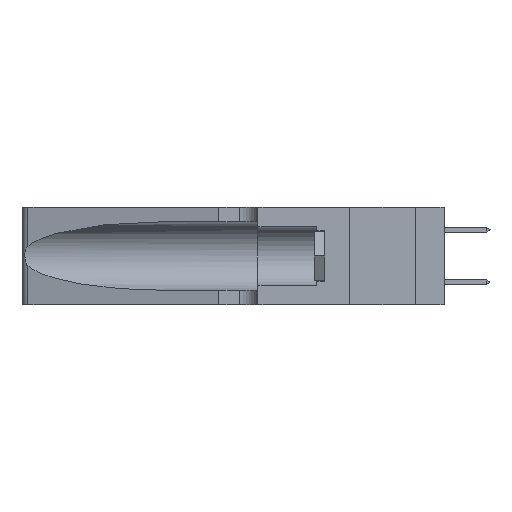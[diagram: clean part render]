
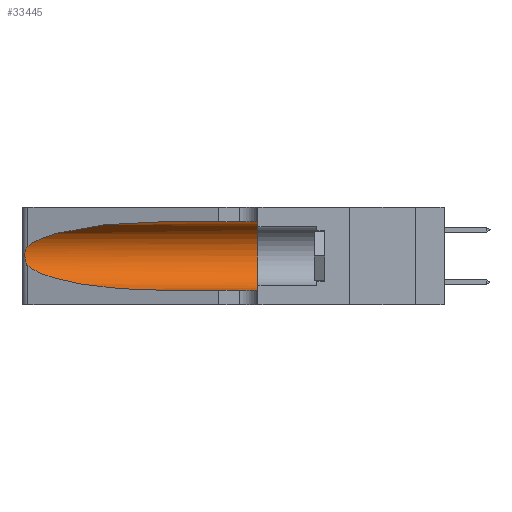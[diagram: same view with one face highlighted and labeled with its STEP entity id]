
A CAD part, left-side view. The second image highlights one B-rep face of the part: STEP entity #33445.
In plain terms, the highlighted cylindrical face has radius 3.308 mm (diameter 6.617 mm), a partial arc.
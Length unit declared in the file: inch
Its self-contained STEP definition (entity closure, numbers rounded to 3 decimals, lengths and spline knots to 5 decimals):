
#1452 = EDGE_LOOP ( 'NONE', ( #8038, #8470, #39785, #21762, #18273, #25114 ) ) ;
#2184 = CARTESIAN_POINT ( 'NONE',  ( 0.1305, 0.72297, 0.05475 ) ) ;
#2196 = CARTESIAN_POINT ( 'NONE',  ( 0.26018, 1.23835, 0.19895 ) ) ;
#3761 = VECTOR ( 'NONE', #10321, 39.37008 ) ;
#4998 = CARTESIAN_POINT ( 'NONE',  ( 0.25487, 1.22718, 0.14631 ) ) ;
#6235 = DIRECTION ( 'NONE',  ( 0., -1., 0. ) ) ;
#6544 = CARTESIAN_POINT ( 'NONE',  ( 0.25487, 1.22718, 0.22369 ) ) ;
#6580 = EDGE_CURVE ( 'NONE', #37651, #11041, #28170, .T. ) ;
#7029 = AXIS2_PLACEMENT_3D ( 'NONE', #22305, #6235, #38997 ) ;
#8038 = ORIENTED_EDGE ( 'NONE', *, *, #25024, .T. ) ;
#8470 = ORIENTED_EDGE ( 'NONE', *, *, #18121, .T. ) ;
#9690 = DIRECTION ( 'NONE',  ( 0., 1., 0. ) ) ;
#10237 = DIRECTION ( 'NONE',  ( 0., -1., 0. ) ) ;
#10321 = DIRECTION ( 'NONE',  ( 0., -1., 0. ) ) ;
#10370 = LINE ( 'NONE', #23724, #3761 ) ;
#11041 = VERTEX_POINT ( 'NONE', #36313 ) ;
#11594 = CARTESIAN_POINT ( 'NONE',  ( 0.18966, 0.96281, 0.31525 ) ) ;
#11728 = CARTESIAN_POINT ( 'NONE',  ( 0.2373, 1.15595, 0.28018 ) ) ;
#12830 = CARTESIAN_POINT ( 'NONE',  ( 0.25639, 1.23186, 0.15144 ) ) ;
#13076 = CARTESIAN_POINT ( 'NONE',  ( 0.1305, 0.35, 0.31525 ) ) ;
#13471 = CARTESIAN_POINT ( 'NONE',  ( 0.25487, 1.22718, 0.14631 ) ) ;
#14084 = CARTESIAN_POINT ( 'NONE',  ( 0.1305, 0.72297, 0.31525 ) ) ;
#14651 = VERTEX_POINT ( 'NONE', #14084 ) ;
#14954 = CARTESIAN_POINT ( 'NONE',  ( 0.25555, 1.22994, 0.2215 ) ) ;
#16225 = CARTESIAN_POINT ( 'NONE',  ( 0.25856, 1.23593, 0.16098 ) ) ;
#16981 =( BOUNDED_CURVE ( )  B_SPLINE_CURVE ( 3, ( #33908, #11594, #11728, #18089 ),
 .UNSPECIFIED., .F., .F. ) 
 B_SPLINE_CURVE_WITH_KNOTS ( ( 4, 4 ),
 ( 1.5708, 2.84003 ),
 .UNSPECIFIED. ) 
 CURVE ( )  GEOMETRIC_REPRESENTATION_ITEM ( )  RATIONAL_B_SPLINE_CURVE ( ( 1., 0.87, 0.87, 1. ) ) 
 REPRESENTATION_ITEM ( '' )  );
#18089 = CARTESIAN_POINT ( 'NONE',  ( 0.25487, 1.22718, 0.22369 ) ) ;
#18121 = EDGE_CURVE ( 'NONE', #35919, #19754, #18804, .T. ) ;
#18208 = CARTESIAN_POINT ( 'NONE',  ( 0.25787, 1.23484, 0.2124 ) ) ;
#18270 = EDGE_CURVE ( 'NONE', #24369, #11041, #10370, .T. ) ;
#18273 = ORIENTED_EDGE ( 'NONE', *, *, #6580, .F. ) ;
#18804 = B_SPLINE_CURVE_WITH_KNOTS ( 'NONE', 3,
 ( #31064, #14954, #37580, #18208, #40958, #2196, #31345, #25821, #38545, #16225, #22707, #12830, #29190, #32452 ),
 .UNSPECIFIED., .F., .F.,
 ( 4, 2, 2, 2, 2, 2, 4 ),
 ( 0., 0.00027, 0.00053, 0.00107, 0.0016, 0.00187, 0.00214 ),
 .UNSPECIFIED. ) ;
#19673 = LINE ( 'NONE', #20536, #27769 ) ;
#19754 = VERTEX_POINT ( 'NONE', #13471 ) ;
#20098 =( BOUNDED_CURVE ( )  B_SPLINE_CURVE ( 3, ( #4998, #21510, #24915, #28138 ),
 .UNSPECIFIED., .F., .T. ) 
 B_SPLINE_CURVE_WITH_KNOTS ( ( 4, 4 ),
 ( 3.44316, 4.71239 ),
 .UNSPECIFIED. ) 
 CURVE ( )  GEOMETRIC_REPRESENTATION_ITEM ( )  RATIONAL_B_SPLINE_CURVE ( ( 1., 0.87, 0.87, 1. ) ) 
 REPRESENTATION_ITEM ( '' )  );
#20536 = CARTESIAN_POINT ( 'NONE',  ( 0.1305, 1.61858, 0.31525 ) ) ;
#21410 = AXIS2_PLACEMENT_3D ( 'NONE', #28442, #9690, #40862 ) ;
#21510 = CARTESIAN_POINT ( 'NONE',  ( 0.2373, 1.15595, 0.08982 ) ) ;
#21762 = ORIENTED_EDGE ( 'NONE', *, *, #18270, .T. ) ;
#22305 = CARTESIAN_POINT ( 'NONE',  ( 0.1305, 1.61858, 0.185 ) ) ;
#22329 = EDGE_CURVE ( 'NONE', #19754, #24369, #20098, .T. ) ;
#22707 = CARTESIAN_POINT ( 'NONE',  ( 0.25789, 1.23486, 0.15765 ) ) ;
#23724 = CARTESIAN_POINT ( 'NONE',  ( 0.1305, 1.61858, 0.05475 ) ) ;
#24369 = VERTEX_POINT ( 'NONE', #2184 ) ;
#24915 = CARTESIAN_POINT ( 'NONE',  ( 0.18966, 0.96281, 0.05475 ) ) ;
#25024 = EDGE_CURVE ( 'NONE', #14651, #35919, #16981, .T. ) ;
#25114 = ORIENTED_EDGE ( 'NONE', *, *, #26198, .F. ) ;
#25821 = CARTESIAN_POINT ( 'NONE',  ( 0.26075, 1.23896, 0.178 ) ) ;
#26198 = EDGE_CURVE ( 'NONE', #14651, #37651, #19673, .T. ) ;
#27769 = VECTOR ( 'NONE', #10237, 39.37008 ) ;
#28138 = CARTESIAN_POINT ( 'NONE',  ( 0.1305, 0.72297, 0.05475 ) ) ;
#28170 = CIRCLE ( 'NONE', #21410, 0.13025 ) ;
#28442 = CARTESIAN_POINT ( 'NONE',  ( 0.1305, 0.35, 0.185 ) ) ;
#29190 = CARTESIAN_POINT ( 'NONE',  ( 0.25555, 1.22993, 0.14849 ) ) ;
#29606 = CYLINDRICAL_SURFACE ( 'NONE', #7029, 0.13025 ) ;
#31064 = CARTESIAN_POINT ( 'NONE',  ( 0.25487, 1.22718, 0.22369 ) ) ;
#31345 = CARTESIAN_POINT ( 'NONE',  ( 0.26075, 1.23896, 0.19203 ) ) ;
#32452 = CARTESIAN_POINT ( 'NONE',  ( 0.25487, 1.22718, 0.14631 ) ) ;
#33445 = ADVANCED_FACE ( 'NONE', ( #40263 ), #29606, .F. ) ;
#33908 = CARTESIAN_POINT ( 'NONE',  ( 0.1305, 0.72297, 0.31525 ) ) ;
#35919 = VERTEX_POINT ( 'NONE', #6544 ) ;
#36313 = CARTESIAN_POINT ( 'NONE',  ( 0.1305, 0.35, 0.05475 ) ) ;
#37580 = CARTESIAN_POINT ( 'NONE',  ( 0.25639, 1.23184, 0.21858 ) ) ;
#37651 = VERTEX_POINT ( 'NONE', #13076 ) ;
#38545 = CARTESIAN_POINT ( 'NONE',  ( 0.26017, 1.23833, 0.17102 ) ) ;
#38997 = DIRECTION ( 'NONE',  ( 0., 0., -1. ) ) ;
#39785 = ORIENTED_EDGE ( 'NONE', *, *, #22329, .T. ) ;
#40263 = FACE_OUTER_BOUND ( 'NONE', #1452, .T. ) ;
#40862 = DIRECTION ( 'NONE',  ( 0., 0., 1. ) ) ;
#40958 = CARTESIAN_POINT ( 'NONE',  ( 0.25854, 1.2359, 0.20912 ) ) ;
